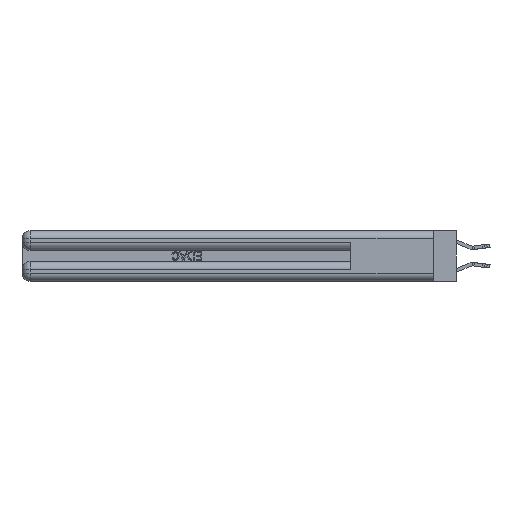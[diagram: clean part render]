
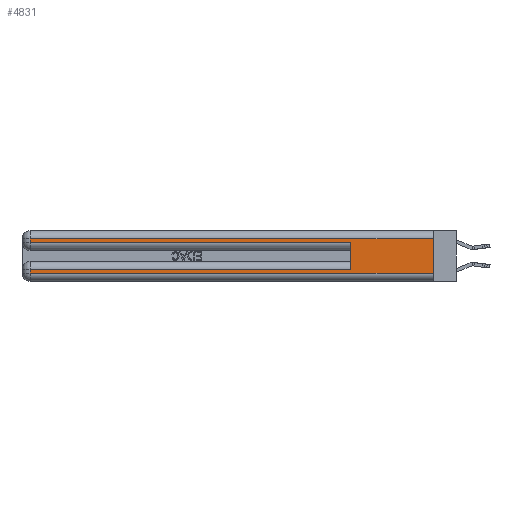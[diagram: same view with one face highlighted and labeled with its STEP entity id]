
A CAD part, left-side view. The second image highlights one B-rep face of the part: STEP entity #4831.
In plain terms, the highlighted planar face has unit normal (-1, 0, 0).
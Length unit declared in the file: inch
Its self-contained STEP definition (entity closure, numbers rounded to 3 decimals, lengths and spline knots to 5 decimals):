
#161 = VERTEX_POINT ( 'NONE', #7290 ) ;
#462 = VECTOR ( 'NONE', #7442, 39.37008 ) ;
#728 = LINE ( 'NONE', #14010, #31557 ) ;
#732 = EDGE_CURVE ( 'NONE', #161, #26528, #728, .T. ) ;
#2497 = ORIENTED_EDGE ( 'NONE', *, *, #22982, .T. ) ;
#2619 = PLANE ( 'NONE',  #29792 ) ;
#2912 = VECTOR ( 'NONE', #31205, 39.37008 ) ;
#4352 = VERTEX_POINT ( 'NONE', #15589 ) ;
#4718 = ORIENTED_EDGE ( 'NONE', *, *, #5185, .T. ) ;
#4800 = LINE ( 'NONE', #23682, #26370 ) ;
#4831 = ADVANCED_FACE ( 'NONE', ( #15906 ), #2619, .F. ) ;
#5185 = EDGE_CURVE ( 'NONE', #24786, #28336, #4800, .T. ) ;
#5673 = ORIENTED_EDGE ( 'NONE', *, *, #732, .F. ) ;
#7290 = CARTESIAN_POINT ( 'NONE',  ( 0., 0.6, 0.085 ) ) ;
#7442 = DIRECTION ( 'NONE',  ( 0., -1., 0. ) ) ;
#7939 = DIRECTION ( 'NONE',  ( 0., 1., 0. ) ) ;
#9486 = ORIENTED_EDGE ( 'NONE', *, *, #22062, .F. ) ;
#10231 = CARTESIAN_POINT ( 'NONE',  ( 0., 0., 0.37 ) ) ;
#10377 = CARTESIAN_POINT ( 'NONE',  ( 0., 2.94, 0.31 ) ) ;
#11017 = LINE ( 'NONE', #13481, #25608 ) ;
#12339 = CARTESIAN_POINT ( 'NONE',  ( 0., 0., 0.06 ) ) ;
#12856 = DIRECTION ( 'NONE',  ( 0., 0., -1. ) ) ;
#13188 = LINE ( 'NONE', #28932, #25861 ) ;
#13481 = CARTESIAN_POINT ( 'NONE',  ( 0., 2.94, 0.37 ) ) ;
#14010 = CARTESIAN_POINT ( 'NONE',  ( 0., 0.6, 0.145 ) ) ;
#14185 = DIRECTION ( 'NONE',  ( 0., 0., 1. ) ) ;
#14355 = DIRECTION ( 'NONE',  ( 0., -1., 0. ) ) ;
#14650 = ORIENTED_EDGE ( 'NONE', *, *, #30124, .T. ) ;
#14987 = VECTOR ( 'NONE', #12856, 39.37008 ) ;
#15002 = ORIENTED_EDGE ( 'NONE', *, *, #30869, .T. ) ;
#15112 = ORIENTED_EDGE ( 'NONE', *, *, #26875, .T. ) ;
#15215 = VERTEX_POINT ( 'NONE', #25592 ) ;
#15589 = CARTESIAN_POINT ( 'NONE',  ( 0., 0., 0.06 ) ) ;
#15635 = DIRECTION ( 'NONE',  ( 0., 0., -1. ) ) ;
#15906 = FACE_OUTER_BOUND ( 'NONE', #16779, .T. ) ;
#16779 = EDGE_LOOP ( 'NONE', ( #9486, #14650, #2497, #15002, #5673, #15112, #4718, #30578 ) ) ;
#17666 = CARTESIAN_POINT ( 'NONE',  ( 0., 0., 0.285 ) ) ;
#18890 = DIRECTION ( 'NONE',  ( 0., 0., -1. ) ) ;
#19747 = EDGE_CURVE ( 'NONE', #28336, #4352, #20731, .T. ) ;
#20513 = LINE ( 'NONE', #28577, #2912 ) ;
#20731 = LINE ( 'NONE', #12339, #462 ) ;
#21080 = CARTESIAN_POINT ( 'NONE',  ( 0., 0.6, 0.285 ) ) ;
#21668 = DIRECTION ( 'NONE',  ( 1., 0., 0. ) ) ;
#22062 = EDGE_CURVE ( 'NONE', #15215, #4352, #32289, .T. ) ;
#22982 = EDGE_CURVE ( 'NONE', #28890, #31110, #11017, .T. ) ;
#23077 = CARTESIAN_POINT ( 'NONE',  ( 0., 0., 0.37 ) ) ;
#23682 = CARTESIAN_POINT ( 'NONE',  ( 0., 2.94, 0.37 ) ) ;
#24786 = VERTEX_POINT ( 'NONE', #30259 ) ;
#25592 = CARTESIAN_POINT ( 'NONE',  ( 0., 0., 0.31 ) ) ;
#25608 = VECTOR ( 'NONE', #18890, 39.37008 ) ;
#25861 = VECTOR ( 'NONE', #7939, 39.37008 ) ;
#26370 = VECTOR ( 'NONE', #15635, 39.37008 ) ;
#26528 = VERTEX_POINT ( 'NONE', #21080 ) ;
#26875 = EDGE_CURVE ( 'NONE', #161, #24786, #20513, .T. ) ;
#26920 = DIRECTION ( 'NONE',  ( 0., 0., -1. ) ) ;
#28336 = VERTEX_POINT ( 'NONE', #34221 ) ;
#28577 = CARTESIAN_POINT ( 'NONE',  ( 0., 0., 0.085 ) ) ;
#28711 = VECTOR ( 'NONE', #14355, 39.37008 ) ;
#28890 = VERTEX_POINT ( 'NONE', #10377 ) ;
#28932 = CARTESIAN_POINT ( 'NONE',  ( 0., 0., 0.31 ) ) ;
#29792 = AXIS2_PLACEMENT_3D ( 'NONE', #23077, #21668, #26920 ) ;
#30124 = EDGE_CURVE ( 'NONE', #15215, #28890, #13188, .T. ) ;
#30259 = CARTESIAN_POINT ( 'NONE',  ( 0., 2.94, 0.085 ) ) ;
#30459 = LINE ( 'NONE', #17666, #28711 ) ;
#30578 = ORIENTED_EDGE ( 'NONE', *, *, #19747, .T. ) ;
#30869 = EDGE_CURVE ( 'NONE', #31110, #26528, #30459, .T. ) ;
#31110 = VERTEX_POINT ( 'NONE', #34456 ) ;
#31205 = DIRECTION ( 'NONE',  ( 0., 1., 0. ) ) ;
#31557 = VECTOR ( 'NONE', #14185, 39.37008 ) ;
#32289 = LINE ( 'NONE', #10231, #14987 ) ;
#34221 = CARTESIAN_POINT ( 'NONE',  ( 0., 2.94, 0.06 ) ) ;
#34456 = CARTESIAN_POINT ( 'NONE',  ( 0., 2.94, 0.285 ) ) ;
